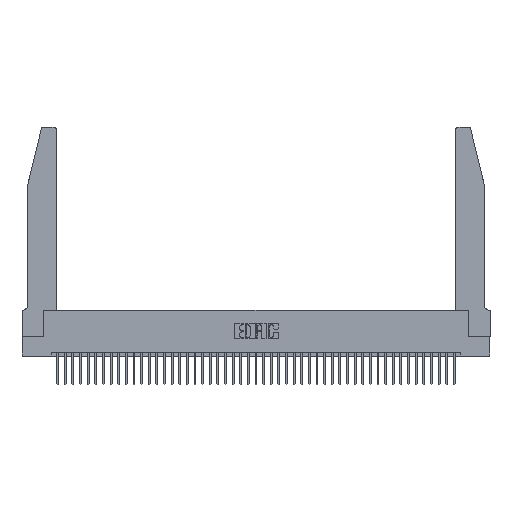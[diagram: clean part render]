
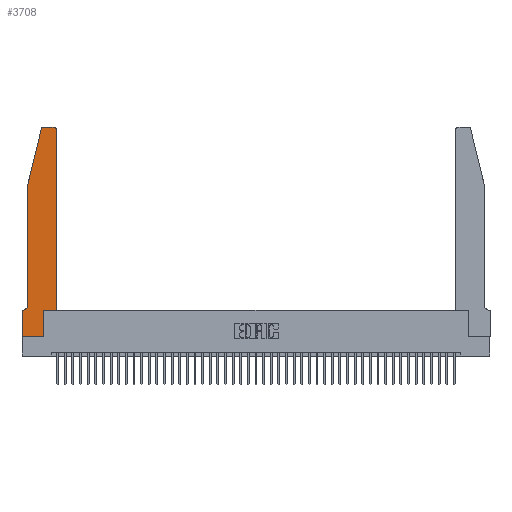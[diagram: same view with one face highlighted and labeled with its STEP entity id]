
A CAD part, top view. The second image highlights one B-rep face of the part: STEP entity #3708.
In plain terms, the highlighted planar face has unit normal (0, 0, 1).
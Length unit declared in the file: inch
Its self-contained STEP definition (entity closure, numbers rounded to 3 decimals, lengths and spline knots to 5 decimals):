
#134 = ORIENTED_EDGE ( 'NONE', *, *, #25668, .T. ) ;
#1150 = DIRECTION ( 'NONE',  ( -1., 0., 0. ) ) ;
#1207 = VECTOR ( 'NONE', #1150, 39.37008 ) ;
#1589 = VECTOR ( 'NONE', #19809, 39.37008 ) ;
#1817 = CARTESIAN_POINT ( 'NONE',  ( 0., 0., 0.37 ) ) ;
#2043 = VERTEX_POINT ( 'NONE', #14949 ) ;
#2146 = ORIENTED_EDGE ( 'NONE', *, *, #21845, .T. ) ;
#2419 = CIRCLE ( 'NONE', #26705, 0.03 ) ;
#2653 = EDGE_CURVE ( 'NONE', #12024, #22010, #10497, .T. ) ;
#3024 = LINE ( 'NONE', #3374, #20533 ) ;
#3374 = CARTESIAN_POINT ( 'NONE',  ( 0.4505, 0.35, 0.37 ) ) ;
#3387 = PLANE ( 'NONE',  #7936 ) ;
#3454 = CARTESIAN_POINT ( 'NONE',  ( 0.0055, 0.42, 0.37 ) ) ;
#3494 = DIRECTION ( 'NONE',  ( 0., -1., 0. ) ) ;
#3708 = ADVANCED_FACE ( 'NONE', ( #21362 ), #3387, .T. ) ;
#3772 = VERTEX_POINT ( 'NONE', #17744 ) ;
#4891 = VERTEX_POINT ( 'NONE', #23897 ) ;
#5214 = LINE ( 'NONE', #7564, #13360 ) ;
#5505 = DIRECTION ( 'NONE',  ( 1., 0., 0. ) ) ;
#6010 = CARTESIAN_POINT ( 'NONE',  ( 0.284, 2.72, 0.37 ) ) ;
#6880 = AXIS2_PLACEMENT_3D ( 'NONE', #3454, #27810, #6947 ) ;
#6947 = DIRECTION ( 'NONE',  ( -1., 0., 0. ) ) ;
#7481 = CARTESIAN_POINT ( 'NONE',  ( 0.2865, 0.35, 0.37 ) ) ;
#7564 = CARTESIAN_POINT ( 'NONE',  ( 0.0755, 2., 0.37 ) ) ;
#7813 = VERTEX_POINT ( 'NONE', #16413 ) ;
#7936 = AXIS2_PLACEMENT_3D ( 'NONE', #31181, #10364, #34624 ) ;
#8833 = CARTESIAN_POINT ( 'NONE',  ( 0.25487, 2.72718, 0.37 ) ) ;
#9198 = DIRECTION ( 'NONE',  ( 0., 1., 0. ) ) ;
#9506 = DIRECTION ( 'NONE',  ( 1., 0., 0. ) ) ;
#10351 = DIRECTION ( 'NONE',  ( 1., 0., 0. ) ) ;
#10364 = DIRECTION ( 'NONE',  ( 0., 0., 1. ) ) ;
#10497 = LINE ( 'NONE', #39201, #1207 ) ;
#10601 = VERTEX_POINT ( 'NONE', #17227 ) ;
#10709 = CARTESIAN_POINT ( 'NONE',  ( 0.0055, 0.35, 0.37 ) ) ;
#11053 = DIRECTION ( 'NONE',  ( 0., -1., 0. ) ) ;
#11770 = ORIENTED_EDGE ( 'NONE', *, *, #13176, .T. ) ;
#11869 = VECTOR ( 'NONE', #16669, 39.37008 ) ;
#12024 = VERTEX_POINT ( 'NONE', #10709 ) ;
#13034 = LINE ( 'NONE', #16240, #1589 ) ;
#13176 = EDGE_CURVE ( 'NONE', #10601, #37512, #5214, .T. ) ;
#13360 = VECTOR ( 'NONE', #11053, 39.37008 ) ;
#14267 = ORIENTED_EDGE ( 'NONE', *, *, #20002, .T. ) ;
#14661 = CIRCLE ( 'NONE', #39196, 0.03 ) ;
#14881 = LINE ( 'NONE', #20383, #24205 ) ;
#14949 = CARTESIAN_POINT ( 'NONE',  ( 0.4505, 2.72, 0.37 ) ) ;
#15336 = ORIENTED_EDGE ( 'NONE', *, *, #2653, .T. ) ;
#15603 = EDGE_CURVE ( 'NONE', #4891, #29630, #26071, .T. ) ;
#16240 = CARTESIAN_POINT ( 'NONE',  ( 0.2605, 2.75, 0.37 ) ) ;
#16306 = ORIENTED_EDGE ( 'NONE', *, *, #33829, .T. ) ;
#16413 = CARTESIAN_POINT ( 'NONE',  ( 0.4205, 2.75, 0.37 ) ) ;
#16477 = EDGE_CURVE ( 'NONE', #22010, #3772, #38335, .T. ) ;
#16669 = DIRECTION ( 'NONE',  ( -0.239, -0.971, 0. ) ) ;
#17227 = CARTESIAN_POINT ( 'NONE',  ( 0.0755, 2., 0.37 ) ) ;
#17587 = ORIENTED_EDGE ( 'NONE', *, *, #44443, .T. ) ;
#17744 = CARTESIAN_POINT ( 'NONE',  ( 0., 0., 0.37 ) ) ;
#18513 = EDGE_CURVE ( 'NONE', #44686, #31739, #2419, .T. ) ;
#19095 = CARTESIAN_POINT ( 'NONE',  ( 0.4205, 2.72, 0.37 ) ) ;
#19379 = CARTESIAN_POINT ( 'NONE',  ( 0.0755, 0.42, 0.37 ) ) ;
#19809 = DIRECTION ( 'NONE',  ( -1., 0., 0. ) ) ;
#20002 = EDGE_CURVE ( 'NONE', #37512, #12024, #25752, .T. ) ;
#20187 = CARTESIAN_POINT ( 'NONE',  ( 0., 0.35, 0.37 ) ) ;
#20228 = CARTESIAN_POINT ( 'NONE',  ( 0.0755, 2., 0.37 ) ) ;
#20383 = CARTESIAN_POINT ( 'NONE',  ( 0.4505, 0.35, 0.37 ) ) ;
#20401 = ORIENTED_EDGE ( 'NONE', *, *, #16477, .T. ) ;
#20533 = VECTOR ( 'NONE', #10351, 39.37008 ) ;
#21362 = FACE_OUTER_BOUND ( 'NONE', #33419, .T. ) ;
#21845 = EDGE_CURVE ( 'NONE', #3772, #4891, #35084, .T. ) ;
#22010 = VERTEX_POINT ( 'NONE', #20187 ) ;
#22575 = DIRECTION ( 'NONE',  ( 1., 0., 0. ) ) ;
#23497 = EDGE_CURVE ( 'NONE', #36555, #2043, #14881, .T. ) ;
#23897 = CARTESIAN_POINT ( 'NONE',  ( 0.2865, 0., 0.37 ) ) ;
#24205 = VECTOR ( 'NONE', #40953, 39.37008 ) ;
#25668 = EDGE_CURVE ( 'NONE', #7813, #44686, #13034, .T. ) ;
#25752 = CIRCLE ( 'NONE', #6880, 0.07 ) ;
#25975 = VECTOR ( 'NONE', #5505, 39.37008 ) ;
#26071 = LINE ( 'NONE', #26708, #42168 ) ;
#26705 = AXIS2_PLACEMENT_3D ( 'NONE', #6010, #30320, #9506 ) ;
#26708 = CARTESIAN_POINT ( 'NONE',  ( 0.2865, 0.35, 0.37 ) ) ;
#27159 = EDGE_CURVE ( 'NONE', #31739, #10601, #31455, .T. ) ;
#27768 = CARTESIAN_POINT ( 'NONE',  ( 0.4505, 0.35, 0.37 ) ) ;
#27810 = DIRECTION ( 'NONE',  ( 0., 0., -1. ) ) ;
#28148 = VECTOR ( 'NONE', #3494, 39.37008 ) ;
#29630 = VERTEX_POINT ( 'NONE', #7481 ) ;
#30320 = DIRECTION ( 'NONE',  ( 0., 0., 1. ) ) ;
#31181 = CARTESIAN_POINT ( 'NONE',  ( 0., 0.35, 0.37 ) ) ;
#31455 = LINE ( 'NONE', #20228, #11869 ) ;
#31739 = VERTEX_POINT ( 'NONE', #8833 ) ;
#33419 = EDGE_LOOP ( 'NONE', ( #134, #42877, #43721, #11770, #14267, #15336, #20401, #2146, #35972, #17587, #41866, #16306 ) ) ;
#33829 = EDGE_CURVE ( 'NONE', #2043, #7813, #14661, .T. ) ;
#34624 = DIRECTION ( 'NONE',  ( 1., 0., 0. ) ) ;
#35084 = LINE ( 'NONE', #1817, #25975 ) ;
#35972 = ORIENTED_EDGE ( 'NONE', *, *, #15603, .T. ) ;
#36336 = CARTESIAN_POINT ( 'NONE',  ( 0., 0., 0.37 ) ) ;
#36555 = VERTEX_POINT ( 'NONE', #27768 ) ;
#37512 = VERTEX_POINT ( 'NONE', #19379 ) ;
#38335 = LINE ( 'NONE', #36336, #28148 ) ;
#39196 = AXIS2_PLACEMENT_3D ( 'NONE', #19095, #43138, #22575 ) ;
#39201 = CARTESIAN_POINT ( 'NONE',  ( 0.0755, 0.35, 0.37 ) ) ;
#39230 = CARTESIAN_POINT ( 'NONE',  ( 0.284, 2.75, 0.37 ) ) ;
#40953 = DIRECTION ( 'NONE',  ( 0., 1., 0. ) ) ;
#41866 = ORIENTED_EDGE ( 'NONE', *, *, #23497, .T. ) ;
#42168 = VECTOR ( 'NONE', #9198, 39.37008 ) ;
#42877 = ORIENTED_EDGE ( 'NONE', *, *, #18513, .T. ) ;
#43138 = DIRECTION ( 'NONE',  ( 0., 0., 1. ) ) ;
#43721 = ORIENTED_EDGE ( 'NONE', *, *, #27159, .T. ) ;
#44443 = EDGE_CURVE ( 'NONE', #29630, #36555, #3024, .T. ) ;
#44686 = VERTEX_POINT ( 'NONE', #39230 ) ;
